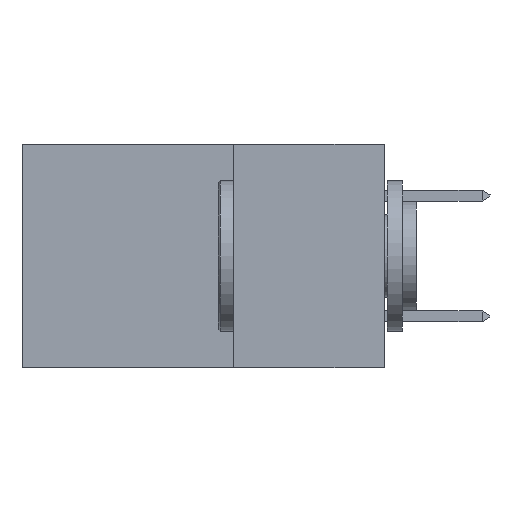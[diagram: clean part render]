
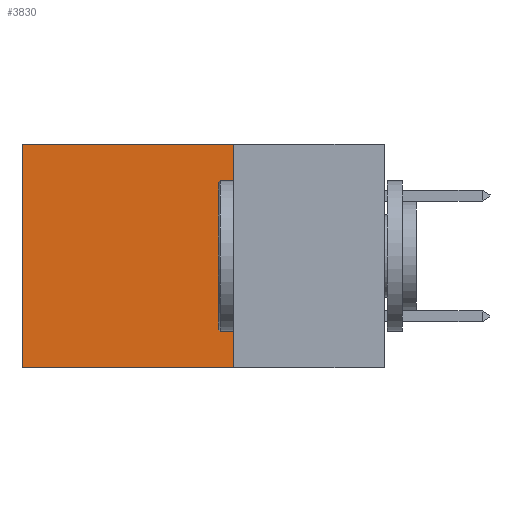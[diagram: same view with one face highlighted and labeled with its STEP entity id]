
A CAD part, left-side view. The second image highlights one B-rep face of the part: STEP entity #3830.
In plain terms, the highlighted planar face has unit normal (-1, 0, 0).
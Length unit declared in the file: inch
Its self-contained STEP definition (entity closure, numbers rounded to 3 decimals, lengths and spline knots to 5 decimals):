
#1210 = CARTESIAN_POINT ( 'NONE',  ( 0.2875, 0.6, 0. ) ) ;
#1627 = ORIENTED_EDGE ( 'NONE', *, *, #6893, .T. ) ;
#3830 = ADVANCED_FACE ( 'NONE', ( #21962 ), #11104, .F. ) ;
#5551 = LINE ( 'NONE', #16558, #20037 ) ;
#5764 = LINE ( 'NONE', #10171, #22311 ) ;
#6893 = EDGE_CURVE ( 'NONE', #27294, #30341, #16521, .T. ) ;
#10171 = CARTESIAN_POINT ( 'NONE',  ( 0.2875, 0.25, -0.37 ) ) ;
#10803 = ORIENTED_EDGE ( 'NONE', *, *, #39883, .F. ) ;
#11104 = PLANE ( 'NONE',  #36921 ) ;
#11711 = EDGE_CURVE ( 'NONE', #13744, #18363, #27548, .T. ) ;
#13744 = VERTEX_POINT ( 'NONE', #19501 ) ;
#16169 = EDGE_LOOP ( 'NONE', ( #1627, #10803, #36401, #21831 ) ) ;
#16521 = LINE ( 'NONE', #28842, #32023 ) ;
#16558 = CARTESIAN_POINT ( 'NONE',  ( 0.2875, 0.25, 0. ) ) ;
#16562 = DIRECTION ( 'NONE',  ( 0., 0., -1. ) ) ;
#18363 = VERTEX_POINT ( 'NONE', #40660 ) ;
#18758 = VECTOR ( 'NONE', #40456, 39.37008 ) ;
#19501 = CARTESIAN_POINT ( 'NONE',  ( 0.2875, 0.25, 0. ) ) ;
#20037 = VECTOR ( 'NONE', #33179, 39.37008 ) ;
#21104 = CARTESIAN_POINT ( 'NONE',  ( 0.2875, 0.25, 0. ) ) ;
#21831 = ORIENTED_EDGE ( 'NONE', *, *, #35595, .T. ) ;
#21962 = FACE_OUTER_BOUND ( 'NONE', #16169, .T. ) ;
#22311 = VECTOR ( 'NONE', #33038, 39.37008 ) ;
#24435 = DIRECTION ( 'NONE',  ( 0., 0., -1. ) ) ;
#27294 = VERTEX_POINT ( 'NONE', #1210 ) ;
#27548 = LINE ( 'NONE', #30665, #18758 ) ;
#28842 = CARTESIAN_POINT ( 'NONE',  ( 0.2875, 0.6, 0. ) ) ;
#30341 = VERTEX_POINT ( 'NONE', #32929 ) ;
#30665 = CARTESIAN_POINT ( 'NONE',  ( 0.2875, 0.25, 0. ) ) ;
#32023 = VECTOR ( 'NONE', #16562, 39.37008 ) ;
#32929 = CARTESIAN_POINT ( 'NONE',  ( 0.2875, 0.6, -0.37 ) ) ;
#33038 = DIRECTION ( 'NONE',  ( 0., 1., 0. ) ) ;
#33179 = DIRECTION ( 'NONE',  ( 0., 1., 0. ) ) ;
#35595 = EDGE_CURVE ( 'NONE', #13744, #27294, #5551, .T. ) ;
#36401 = ORIENTED_EDGE ( 'NONE', *, *, #11711, .F. ) ;
#36921 = AXIS2_PLACEMENT_3D ( 'NONE', #21104, #37428, #24435 ) ;
#37428 = DIRECTION ( 'NONE',  ( 1., 0., 0. ) ) ;
#39883 = EDGE_CURVE ( 'NONE', #18363, #30341, #5764, .T. ) ;
#40456 = DIRECTION ( 'NONE',  ( 0., 0., -1. ) ) ;
#40660 = CARTESIAN_POINT ( 'NONE',  ( 0.2875, 0.25, -0.37 ) ) ;
